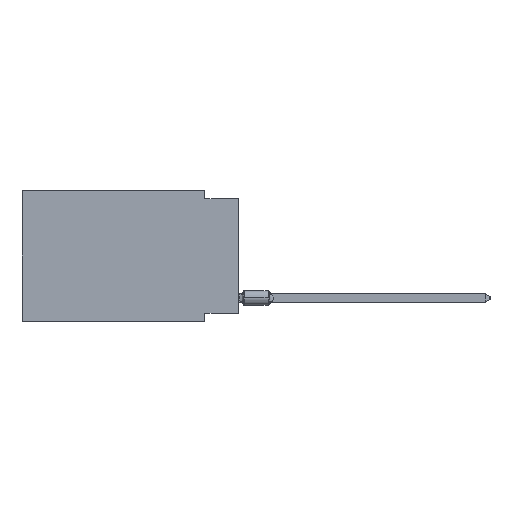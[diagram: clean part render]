
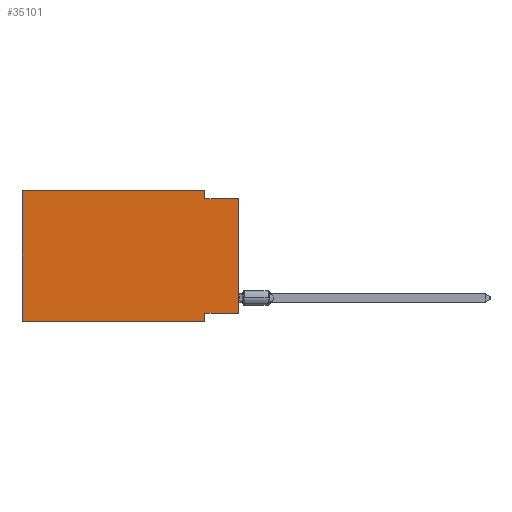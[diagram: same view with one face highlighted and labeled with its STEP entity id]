
A CAD part, left-side view. The second image highlights one B-rep face of the part: STEP entity #35101.
In plain terms, the highlighted planar face has unit normal (-1, 0, 0).
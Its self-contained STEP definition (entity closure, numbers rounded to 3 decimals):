
#981 = CARTESIAN_POINT ( 'NONE',  ( 0., 2.54, -0.635 ) ) ;
#2123 = VECTOR ( 'NONE', #22196, 1000. ) ;
#2443 = VECTOR ( 'NONE', #21785, 1000. ) ;
#3817 = CARTESIAN_POINT ( 'NONE',  ( 0., 0., -9.271 ) ) ;
#4019 = ORIENTED_EDGE ( 'NONE', *, *, #28709, .F. ) ;
#4434 = LINE ( 'NONE', #15977, #5070 ) ;
#4908 = DIRECTION ( 'NONE',  ( 1., 0., 0. ) ) ;
#5070 = VECTOR ( 'NONE', #10490, 1000. ) ;
#5092 = FACE_OUTER_BOUND ( 'NONE', #31225, .T. ) ;
#6471 = CARTESIAN_POINT ( 'NONE',  ( 0., 16.383, 0. ) ) ;
#6571 = LINE ( 'NONE', #21324, #7626 ) ;
#6657 = EDGE_CURVE ( 'NONE', #8246, #21662, #15588, .T. ) ;
#6671 = LINE ( 'NONE', #6471, #30482 ) ;
#7626 = VECTOR ( 'NONE', #35896, 1000. ) ;
#7767 = CARTESIAN_POINT ( 'NONE',  ( 0., 2.54, 0. ) ) ;
#7781 = EDGE_CURVE ( 'NONE', #20169, #27597, #6571, .T. ) ;
#7919 = CARTESIAN_POINT ( 'NONE',  ( 0., 2.54, -9.906 ) ) ;
#8246 = VERTEX_POINT ( 'NONE', #16508 ) ;
#10250 = CARTESIAN_POINT ( 'NONE',  ( 0., 2.54, 0. ) ) ;
#10490 = DIRECTION ( 'NONE',  ( 0., 0., 1. ) ) ;
#11921 = VECTOR ( 'NONE', #23703, 1000. ) ;
#13129 = CARTESIAN_POINT ( 'NONE',  ( 0., 0., -0.635 ) ) ;
#13130 = EDGE_CURVE ( 'NONE', #14735, #33149, #30541, .T. ) ;
#14202 = ORIENTED_EDGE ( 'NONE', *, *, #35992, .F. ) ;
#14474 = ORIENTED_EDGE ( 'NONE', *, *, #32003, .F. ) ;
#14735 = VERTEX_POINT ( 'NONE', #981 ) ;
#15588 = LINE ( 'NONE', #21647, #2123 ) ;
#15895 = LINE ( 'NONE', #10250, #2443 ) ;
#15977 = CARTESIAN_POINT ( 'NONE',  ( 0., 0., 0. ) ) ;
#16203 = CARTESIAN_POINT ( 'NONE',  ( 0., 0., -0.635 ) ) ;
#16454 = DIRECTION ( 'NONE',  ( 0., 0., -1. ) ) ;
#16508 = CARTESIAN_POINT ( 'NONE',  ( 0., 16.383, -9.906 ) ) ;
#16970 = VERTEX_POINT ( 'NONE', #28612 ) ;
#18643 = VECTOR ( 'NONE', #21671, 1000. ) ;
#19666 = CARTESIAN_POINT ( 'NONE',  ( 0., 16.383, 0. ) ) ;
#20169 = VERTEX_POINT ( 'NONE', #25303 ) ;
#20284 = DIRECTION ( 'NONE',  ( 0., -1., 0. ) ) ;
#21084 = ORIENTED_EDGE ( 'NONE', *, *, #25630, .T. ) ;
#21240 = LINE ( 'NONE', #3817, #11921 ) ;
#21324 = CARTESIAN_POINT ( 'NONE',  ( 0., 2.54, -9.906 ) ) ;
#21647 = CARTESIAN_POINT ( 'NONE',  ( 0., 16.383, 0. ) ) ;
#21662 = VERTEX_POINT ( 'NONE', #36754 ) ;
#21671 = DIRECTION ( 'NONE',  ( 0., -1., 0. ) ) ;
#21785 = DIRECTION ( 'NONE',  ( 0., 0., -1. ) ) ;
#21844 = DIRECTION ( 'NONE',  ( 0., -1., 0. ) ) ;
#22196 = DIRECTION ( 'NONE',  ( 0., 0., 1. ) ) ;
#22801 = ORIENTED_EDGE ( 'NONE', *, *, #7781, .F. ) ;
#23096 = ORIENTED_EDGE ( 'NONE', *, *, #36496, .T. ) ;
#23703 = DIRECTION ( 'NONE',  ( 0., 1., 0. ) ) ;
#23767 = ORIENTED_EDGE ( 'NONE', *, *, #6657, .F. ) ;
#24701 = LINE ( 'NONE', #33035, #18643 ) ;
#25303 = CARTESIAN_POINT ( 'NONE',  ( 0., 2.54, -9.271 ) ) ;
#25588 = AXIS2_PLACEMENT_3D ( 'NONE', #19666, #4908, #16454 ) ;
#25630 = EDGE_CURVE ( 'NONE', #16970, #33149, #4434, .T. ) ;
#26067 = ORIENTED_EDGE ( 'NONE', *, *, #13130, .F. ) ;
#27597 = VERTEX_POINT ( 'NONE', #7919 ) ;
#28612 = CARTESIAN_POINT ( 'NONE',  ( 0., 0., -9.271 ) ) ;
#28709 = EDGE_CURVE ( 'NONE', #16970, #20169, #21240, .T. ) ;
#28841 = VERTEX_POINT ( 'NONE', #7767 ) ;
#30482 = VECTOR ( 'NONE', #20284, 1000. ) ;
#30541 = LINE ( 'NONE', #13129, #32142 ) ;
#30853 = PLANE ( 'NONE',  #25588 ) ;
#31225 = EDGE_LOOP ( 'NONE', ( #21084, #26067, #14474, #14202, #23767, #23096, #22801, #4019 ) ) ;
#32003 = EDGE_CURVE ( 'NONE', #28841, #14735, #15895, .T. ) ;
#32142 = VECTOR ( 'NONE', #21844, 1000. ) ;
#33035 = CARTESIAN_POINT ( 'NONE',  ( 0., 16.383, -9.906 ) ) ;
#33149 = VERTEX_POINT ( 'NONE', #16203 ) ;
#35101 = ADVANCED_FACE ( 'NONE', ( #5092 ), #30853, .F. ) ;
#35896 = DIRECTION ( 'NONE',  ( 0., 0., -1. ) ) ;
#35992 = EDGE_CURVE ( 'NONE', #21662, #28841, #6671, .T. ) ;
#36496 = EDGE_CURVE ( 'NONE', #8246, #27597, #24701, .T. ) ;
#36754 = CARTESIAN_POINT ( 'NONE',  ( 0., 16.383, 0. ) ) ;
